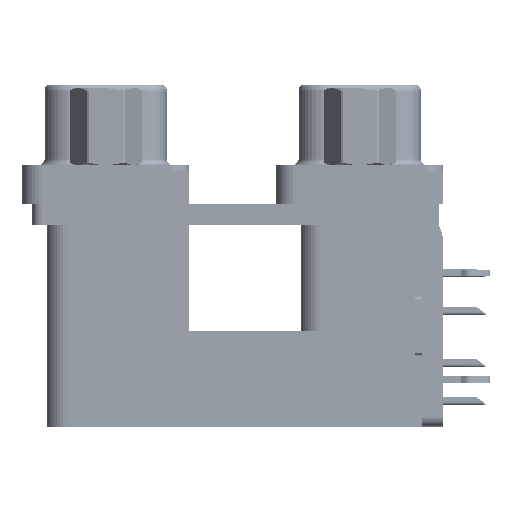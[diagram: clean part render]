
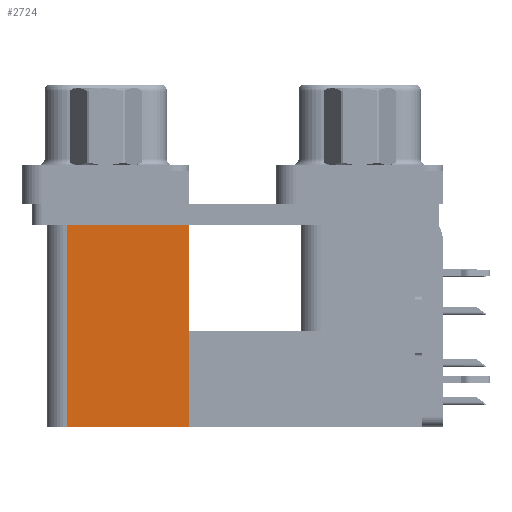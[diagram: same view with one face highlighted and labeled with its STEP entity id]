
A CAD part, left-side view. The second image highlights one B-rep face of the part: STEP entity #2724.
In plain terms, the highlighted planar face has unit normal (-1, 0, 0).
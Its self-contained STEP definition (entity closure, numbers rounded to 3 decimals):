
#2724 = ADVANCED_FACE ( 'NONE', ( #41020 ), #4433, .F. ) ;
#4433 = PLANE ( 'NONE',  #26986 ) ;
#5626 = CARTESIAN_POINT ( 'NONE',  ( 3.79, 12.775, -19.2 ) ) ;
#6893 = DIRECTION ( 'NONE',  ( 0., 1., 0. ) ) ;
#8451 = EDGE_CURVE ( 'NONE', #34811, #46556, #40511, .T. ) ;
#9724 = ORIENTED_EDGE ( 'NONE', *, *, #8451, .F. ) ;
#11567 = ORIENTED_EDGE ( 'NONE', *, *, #41165, .F. ) ;
#11827 = LINE ( 'NONE', #30414, #31136 ) ;
#12690 = CARTESIAN_POINT ( 'NONE',  ( 3.79, 21.975, -2.5 ) ) ;
#14173 = CARTESIAN_POINT ( 'NONE',  ( 3.79, 12.775, -19.2 ) ) ;
#14458 = DIRECTION ( 'NONE',  ( 0., 0., -1. ) ) ;
#17513 = LINE ( 'NONE', #35509, #55110 ) ;
#25609 = VERTEX_POINT ( 'NONE', #12690 ) ;
#26405 = EDGE_LOOP ( 'NONE', ( #32507, #11567, #9724, #34715 ) ) ;
#26986 = AXIS2_PLACEMENT_3D ( 'NONE', #14173, #41316, #14458 ) ;
#28956 = CARTESIAN_POINT ( 'NONE',  ( 3.79, 21.975, -19.2 ) ) ;
#29350 = LINE ( 'NONE', #47322, #41222 ) ;
#30414 = CARTESIAN_POINT ( 'NONE',  ( 3.79, 21.975, -19.2 ) ) ;
#31136 = VECTOR ( 'NONE', #48378, 1000. ) ;
#31262 = EDGE_CURVE ( 'NONE', #34811, #53601, #17513, .T. ) ;
#32507 = ORIENTED_EDGE ( 'NONE', *, *, #52559, .T. ) ;
#34715 = ORIENTED_EDGE ( 'NONE', *, *, #31262, .T. ) ;
#34811 = VERTEX_POINT ( 'NONE', #5626 ) ;
#35509 = CARTESIAN_POINT ( 'NONE',  ( 3.79, 12.775, -19.2 ) ) ;
#39052 = DIRECTION ( 'NONE',  ( 0., 0., 1. ) ) ;
#39926 = DIRECTION ( 'NONE',  ( 0., 1., 0. ) ) ;
#40511 = LINE ( 'NONE', #57594, #56505 ) ;
#41020 = FACE_OUTER_BOUND ( 'NONE', #26405, .T. ) ;
#41165 = EDGE_CURVE ( 'NONE', #46556, #25609, #11827, .T. ) ;
#41222 = VECTOR ( 'NONE', #6893, 1000. ) ;
#41316 = DIRECTION ( 'NONE',  ( 1., 0., 0. ) ) ;
#46556 = VERTEX_POINT ( 'NONE', #28956 ) ;
#47322 = CARTESIAN_POINT ( 'NONE',  ( 3.79, 12.775, -2.5 ) ) ;
#48378 = DIRECTION ( 'NONE',  ( 0., 0., 1. ) ) ;
#52559 = EDGE_CURVE ( 'NONE', #53601, #25609, #29350, .T. ) ;
#53601 = VERTEX_POINT ( 'NONE', #55703 ) ;
#55110 = VECTOR ( 'NONE', #39052, 1000. ) ;
#55703 = CARTESIAN_POINT ( 'NONE',  ( 3.79, 12.775, -2.5 ) ) ;
#56505 = VECTOR ( 'NONE', #39926, 1000. ) ;
#57594 = CARTESIAN_POINT ( 'NONE',  ( 3.79, 12.775, -19.2 ) ) ;
